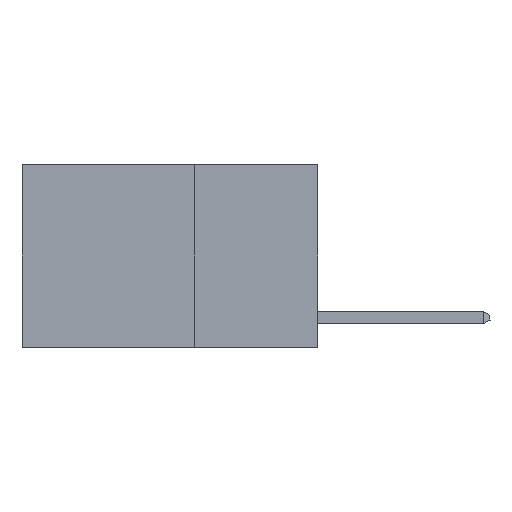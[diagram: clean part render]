
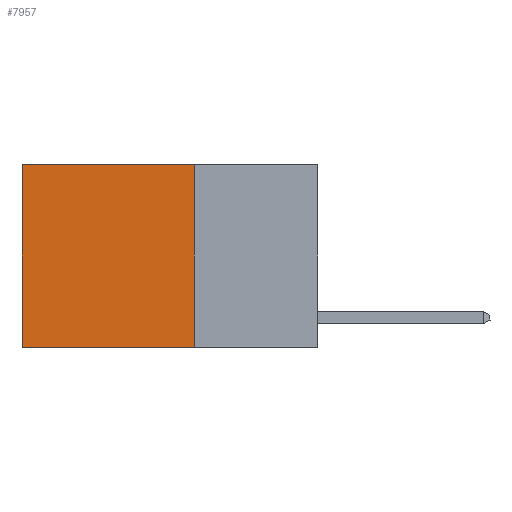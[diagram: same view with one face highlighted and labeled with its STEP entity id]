
A CAD part, left-side view. The second image highlights one B-rep face of the part: STEP entity #7957.
In plain terms, the highlighted planar face has unit normal (-1, 0, 0).
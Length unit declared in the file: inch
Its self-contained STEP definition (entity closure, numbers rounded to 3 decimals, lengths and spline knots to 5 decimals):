
#624 = VECTOR ( 'NONE', #6164, 39.37008 ) ;
#833 = LINE ( 'NONE', #8521, #4555 ) ;
#893 = LINE ( 'NONE', #9567, #624 ) ;
#1193 = EDGE_CURVE ( 'NONE', #7273, #8406, #833, .T. ) ;
#1550 = ORIENTED_EDGE ( 'NONE', *, *, #1193, .F. ) ;
#1696 = VECTOR ( 'NONE', #5456, 39.37008 ) ;
#1725 = EDGE_CURVE ( 'NONE', #4842, #8406, #5775, .T. ) ;
#1784 = AXIS2_PLACEMENT_3D ( 'NONE', #9082, #3396, #8425 ) ;
#2098 = LINE ( 'NONE', #4434, #5902 ) ;
#3396 = DIRECTION ( 'NONE',  ( 1., 0., 0. ) ) ;
#3892 = ORIENTED_EDGE ( 'NONE', *, *, #4459, .T. ) ;
#4434 = CARTESIAN_POINT ( 'NONE',  ( 0.2625, 0.25, 0. ) ) ;
#4459 = EDGE_CURVE ( 'NONE', #6372, #4842, #2098, .T. ) ;
#4555 = VECTOR ( 'NONE', #9434, 39.37008 ) ;
#4842 = VERTEX_POINT ( 'NONE', #7658 ) ;
#4943 = EDGE_LOOP ( 'NONE', ( #7487, #1550, #7176, #3892 ) ) ;
#5192 = FACE_OUTER_BOUND ( 'NONE', #4943, .T. ) ;
#5428 = CARTESIAN_POINT ( 'NONE',  ( 0.2625, 0.6, 0. ) ) ;
#5456 = DIRECTION ( 'NONE',  ( 0., 0., -1. ) ) ;
#5477 = CARTESIAN_POINT ( 'NONE',  ( 0.2625, 0.6, -0.37 ) ) ;
#5775 = LINE ( 'NONE', #5428, #1696 ) ;
#5902 = VECTOR ( 'NONE', #7322, 39.37008 ) ;
#6164 = DIRECTION ( 'NONE',  ( 0., 0., -1. ) ) ;
#6372 = VERTEX_POINT ( 'NONE', #8455 ) ;
#7176 = ORIENTED_EDGE ( 'NONE', *, *, #8403, .F. ) ;
#7273 = VERTEX_POINT ( 'NONE', #8328 ) ;
#7322 = DIRECTION ( 'NONE',  ( 0., 1., 0. ) ) ;
#7487 = ORIENTED_EDGE ( 'NONE', *, *, #1725, .T. ) ;
#7658 = CARTESIAN_POINT ( 'NONE',  ( 0.2625, 0.6, 0. ) ) ;
#7754 = PLANE ( 'NONE',  #1784 ) ;
#7957 = ADVANCED_FACE ( 'NONE', ( #5192 ), #7754, .F. ) ;
#8328 = CARTESIAN_POINT ( 'NONE',  ( 0.2625, 0.25, -0.37 ) ) ;
#8403 = EDGE_CURVE ( 'NONE', #6372, #7273, #893, .T. ) ;
#8406 = VERTEX_POINT ( 'NONE', #5477 ) ;
#8425 = DIRECTION ( 'NONE',  ( 0., 0., -1. ) ) ;
#8455 = CARTESIAN_POINT ( 'NONE',  ( 0.2625, 0.25, 0. ) ) ;
#8521 = CARTESIAN_POINT ( 'NONE',  ( 0.2625, 0.25, -0.37 ) ) ;
#9082 = CARTESIAN_POINT ( 'NONE',  ( 0.2625, 0.25, 0. ) ) ;
#9434 = DIRECTION ( 'NONE',  ( 0., 1., 0. ) ) ;
#9567 = CARTESIAN_POINT ( 'NONE',  ( 0.2625, 0.25, 0. ) ) ;
